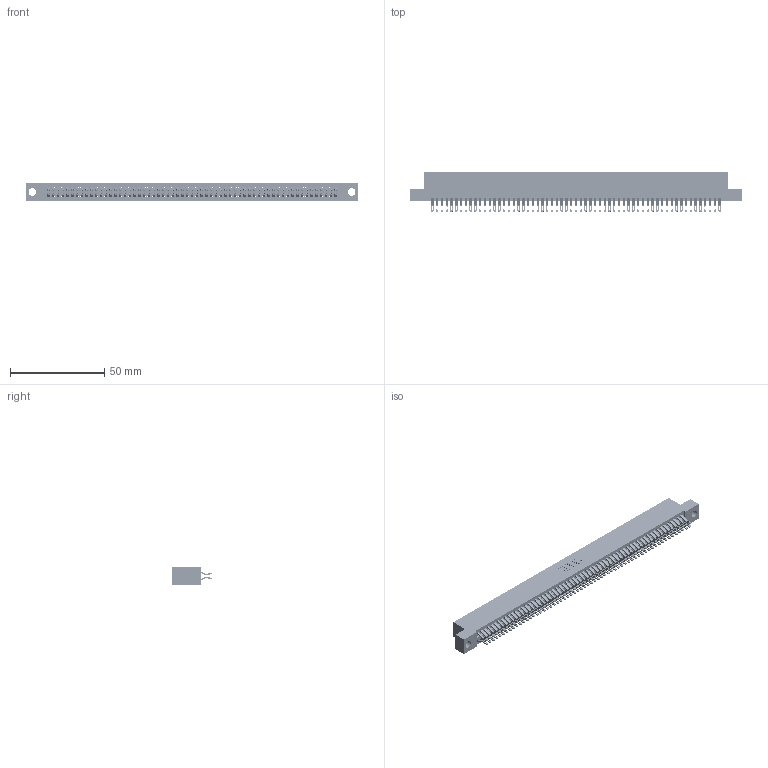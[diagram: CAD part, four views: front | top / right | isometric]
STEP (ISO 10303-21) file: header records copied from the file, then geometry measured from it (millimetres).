
FILE_DESCRIPTION (( 'STEP AP203' ), '1' );
FILE_NAME ('395-122-555-204.STEP', '2018-12-03T19:28:01', ( '' ), ( '' ), 'SwSTEP 2.0', 'SolidWorks 2016', '' );
FILE_SCHEMA (( 'CONFIG_CONTROL_DESIGN' ));
Length unit declared in the file: inch
Products named in the file (3): 395-122-555-204; 345-292-001_555 Tail; 345 Part_Flush Mounting Lugs - 0.156 Dia-TH
Assembly tree (123 placements, depth 2):
  395-122-555-204
    345 Part_Flush Mounting Lugs - 0.156 Dia-TH
    345-292-001_555 Tail  x122
Bounding box: 176.15 x 21.13 x 9.4 mm (x, y, z)
Volume: 17553.7 mm3; surface area: 27361.2 mm2
Topology: 123 solids, 123 shells, 6958 faces, 21935 edges, 14622 vertices
Faces by surface type: plane 3862, cylinder 3096
Entity records: 45633 total; most frequent: CARTESIAN_POINT 7666, ORIENTED_EDGE 7570, DIRECTION 6705, EDGE_CURVE 3785, LINE 3389, VECTOR 3389, VERTEX_POINT 2522, AXIS2_PLACEMENT_3D 1658
